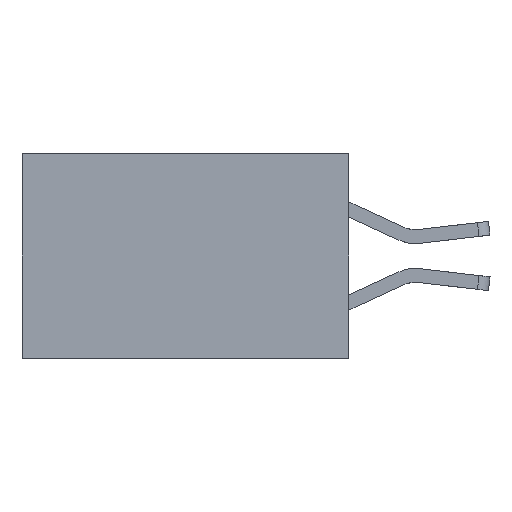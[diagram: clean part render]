
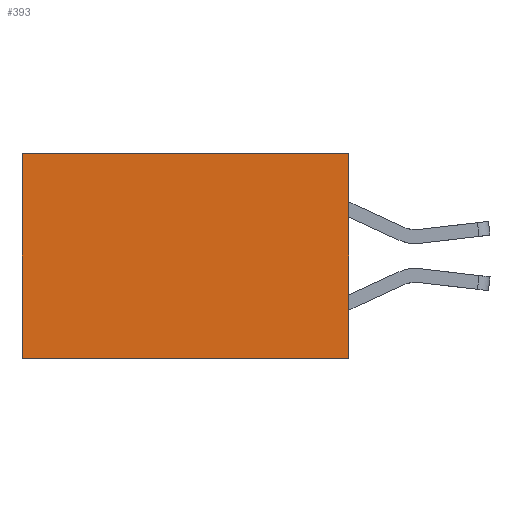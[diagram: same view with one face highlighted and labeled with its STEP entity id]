
A CAD part, left-side view. The second image highlights one B-rep face of the part: STEP entity #393.
In plain terms, the highlighted planar face has unit normal (-1, 0, 0).
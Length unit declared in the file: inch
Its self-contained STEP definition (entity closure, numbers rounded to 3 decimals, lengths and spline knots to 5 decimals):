
#16 = CARTESIAN_POINT ( 'NONE',  ( 0.277, 0., -0.37 ) ) ;
#393 = ADVANCED_FACE ( 'NONE', ( #11441 ), #13316, .F. ) ;
#516 = ORIENTED_EDGE ( 'NONE', *, *, #14263, .T. ) ;
#610 = EDGE_CURVE ( 'NONE', #5590, #14056, #9906, .T. ) ;
#665 = DIRECTION ( 'NONE',  ( 0., 0., -1. ) ) ;
#786 = VECTOR ( 'NONE', #13701, 39.37008 ) ;
#846 = CARTESIAN_POINT ( 'NONE',  ( 0.277, 0., -0.37 ) ) ;
#1494 = EDGE_CURVE ( 'NONE', #10838, #14056, #2850, .T. ) ;
#2055 = ORIENTED_EDGE ( 'NONE', *, *, #13128, .F. ) ;
#2397 = VECTOR ( 'NONE', #2697, 39.37008 ) ;
#2697 = DIRECTION ( 'NONE',  ( 0., 1., 0. ) ) ;
#2740 = CARTESIAN_POINT ( 'NONE',  ( 0.277, 0., 0. ) ) ;
#2850 = LINE ( 'NONE', #14564, #8804 ) ;
#3441 = AXIS2_PLACEMENT_3D ( 'NONE', #5529, #10121, #9379 ) ;
#5529 = CARTESIAN_POINT ( 'NONE',  ( 0.277, 0., -0.37 ) ) ;
#5590 = VERTEX_POINT ( 'NONE', #16 ) ;
#6840 = LINE ( 'NONE', #846, #14591 ) ;
#6954 = CARTESIAN_POINT ( 'NONE',  ( 0.277, 0.59, -0.37 ) ) ;
#8804 = VECTOR ( 'NONE', #665, 39.37008 ) ;
#9050 = CARTESIAN_POINT ( 'NONE',  ( 0.277, 0.59, 0. ) ) ;
#9143 = EDGE_LOOP ( 'NONE', ( #13663, #9652, #2055, #516 ) ) ;
#9379 = DIRECTION ( 'NONE',  ( 0., 0., -1. ) ) ;
#9652 = ORIENTED_EDGE ( 'NONE', *, *, #610, .F. ) ;
#9878 = CARTESIAN_POINT ( 'NONE',  ( 0.277, 0., -0.37 ) ) ;
#9906 = LINE ( 'NONE', #9878, #786 ) ;
#9975 = DIRECTION ( 'NONE',  ( 0., 0., -1. ) ) ;
#10121 = DIRECTION ( 'NONE',  ( 1., 0., 0. ) ) ;
#10838 = VERTEX_POINT ( 'NONE', #9050 ) ;
#11441 = FACE_OUTER_BOUND ( 'NONE', #9143, .T. ) ;
#12942 = CARTESIAN_POINT ( 'NONE',  ( 0.277, 0., 0. ) ) ;
#12959 = VERTEX_POINT ( 'NONE', #12942 ) ;
#13128 = EDGE_CURVE ( 'NONE', #12959, #5590, #6840, .T. ) ;
#13316 = PLANE ( 'NONE',  #3441 ) ;
#13663 = ORIENTED_EDGE ( 'NONE', *, *, #1494, .T. ) ;
#13701 = DIRECTION ( 'NONE',  ( 0., 1., 0. ) ) ;
#14056 = VERTEX_POINT ( 'NONE', #6954 ) ;
#14263 = EDGE_CURVE ( 'NONE', #12959, #10838, #14558, .T. ) ;
#14558 = LINE ( 'NONE', #2740, #2397 ) ;
#14564 = CARTESIAN_POINT ( 'NONE',  ( 0.277, 0.59, -0.37 ) ) ;
#14591 = VECTOR ( 'NONE', #9975, 39.37008 ) ;
